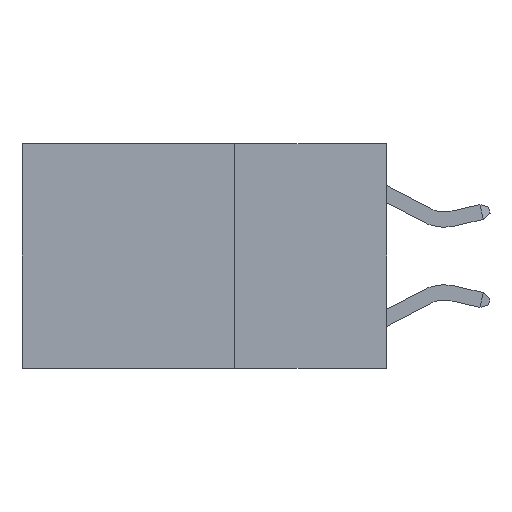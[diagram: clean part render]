
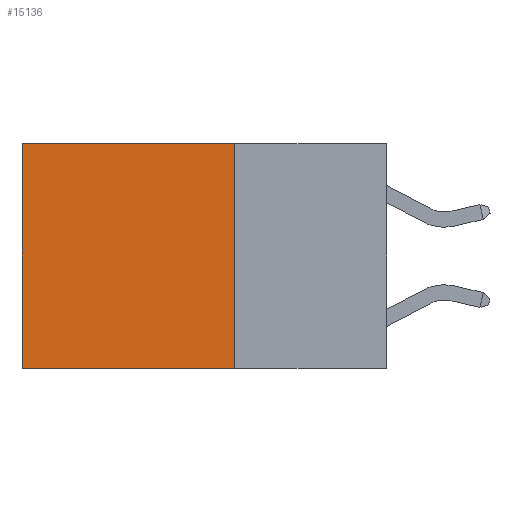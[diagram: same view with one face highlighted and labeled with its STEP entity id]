
A CAD part, left-side view. The second image highlights one B-rep face of the part: STEP entity #15136.
In plain terms, the highlighted planar face has unit normal (-1, 0, 0).
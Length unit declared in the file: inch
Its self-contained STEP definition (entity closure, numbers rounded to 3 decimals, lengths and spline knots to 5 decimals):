
#1424 = LINE ( 'NONE', #25646, #22526 ) ;
#1687 = EDGE_CURVE ( 'NONE', #22932, #6174, #6429, .T. ) ;
#1777 = DIRECTION ( 'NONE',  ( 0., 0., -1. ) ) ;
#3005 = CARTESIAN_POINT ( 'NONE',  ( 0.2625, 0.25, -0.37 ) ) ;
#3375 = LINE ( 'NONE', #8947, #23650 ) ;
#4841 = VECTOR ( 'NONE', #17105, 39.37008 ) ;
#4901 = DIRECTION ( 'NONE',  ( 0., 1., 0. ) ) ;
#6079 = FACE_OUTER_BOUND ( 'NONE', #11545, .T. ) ;
#6174 = VERTEX_POINT ( 'NONE', #22819 ) ;
#6234 = LINE ( 'NONE', #13924, #14716 ) ;
#6316 = CARTESIAN_POINT ( 'NONE',  ( 0.2625, 0.25, 0. ) ) ;
#6429 = LINE ( 'NONE', #3005, #4841 ) ;
#6655 = CARTESIAN_POINT ( 'NONE',  ( 0.2625, 0.25, -0.37 ) ) ;
#8947 = CARTESIAN_POINT ( 'NONE',  ( 0.2625, 0.25, 0. ) ) ;
#8962 = CARTESIAN_POINT ( 'NONE',  ( 0.2625, 0.25, 0. ) ) ;
#10115 = ORIENTED_EDGE ( 'NONE', *, *, #17799, .T. ) ;
#11545 = EDGE_LOOP ( 'NONE', ( #10115, #20896, #19385, #20069 ) ) ;
#11626 = AXIS2_PLACEMENT_3D ( 'NONE', #8962, #15197, #13113 ) ;
#13113 = DIRECTION ( 'NONE',  ( 0., 0., -1. ) ) ;
#13924 = CARTESIAN_POINT ( 'NONE',  ( 0.2625, 0.6, 0. ) ) ;
#14243 = VERTEX_POINT ( 'NONE', #20421 ) ;
#14716 = VECTOR ( 'NONE', #1777, 39.37008 ) ;
#15136 = ADVANCED_FACE ( 'NONE', ( #6079 ), #21357, .F. ) ;
#15197 = DIRECTION ( 'NONE',  ( 1., 0., 0. ) ) ;
#17105 = DIRECTION ( 'NONE',  ( 0., 1., 0. ) ) ;
#17799 = EDGE_CURVE ( 'NONE', #14243, #6174, #6234, .T. ) ;
#19346 = DIRECTION ( 'NONE',  ( 0., 0., -1. ) ) ;
#19385 = ORIENTED_EDGE ( 'NONE', *, *, #23715, .F. ) ;
#20069 = ORIENTED_EDGE ( 'NONE', *, *, #21607, .T. ) ;
#20421 = CARTESIAN_POINT ( 'NONE',  ( 0.2625, 0.6, 0. ) ) ;
#20896 = ORIENTED_EDGE ( 'NONE', *, *, #1687, .F. ) ;
#21357 = PLANE ( 'NONE',  #11626 ) ;
#21607 = EDGE_CURVE ( 'NONE', #22465, #14243, #3375, .T. ) ;
#22465 = VERTEX_POINT ( 'NONE', #6316 ) ;
#22526 = VECTOR ( 'NONE', #19346, 39.37008 ) ;
#22819 = CARTESIAN_POINT ( 'NONE',  ( 0.2625, 0.6, -0.37 ) ) ;
#22932 = VERTEX_POINT ( 'NONE', #6655 ) ;
#23650 = VECTOR ( 'NONE', #4901, 39.37008 ) ;
#23715 = EDGE_CURVE ( 'NONE', #22465, #22932, #1424, .T. ) ;
#25646 = CARTESIAN_POINT ( 'NONE',  ( 0.2625, 0.25, 0. ) ) ;
